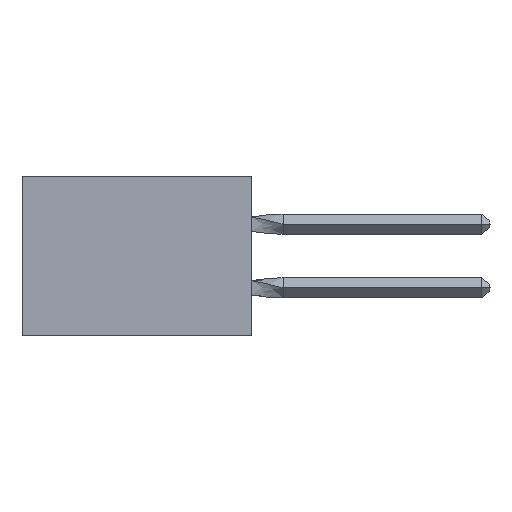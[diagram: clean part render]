
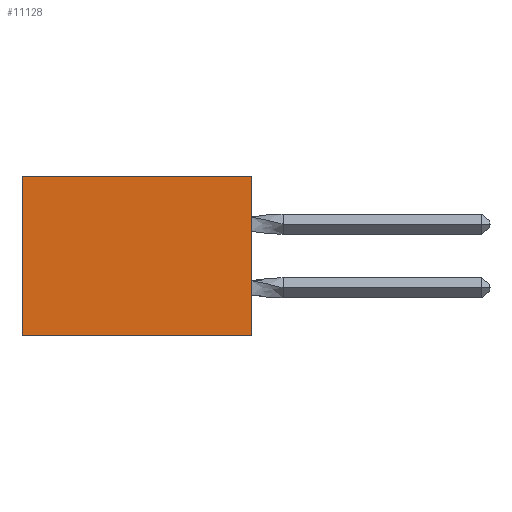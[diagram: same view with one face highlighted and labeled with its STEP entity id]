
A CAD part, left-side view. The second image highlights one B-rep face of the part: STEP entity #11128.
In plain terms, the highlighted planar face has unit normal (-1, 0, 0).
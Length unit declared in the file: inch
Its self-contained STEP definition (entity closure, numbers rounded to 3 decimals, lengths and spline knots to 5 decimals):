
#787 = CARTESIAN_POINT ( 'NONE',  ( 0.305, 0.72, -0.5 ) ) ;
#1518 = CARTESIAN_POINT ( 'NONE',  ( 0.305, 0.72, 0. ) ) ;
#1751 = EDGE_CURVE ( 'NONE', #24773, #32293, #24246, .T. ) ;
#1872 = CARTESIAN_POINT ( 'NONE',  ( 0.305, 0., -0.5 ) ) ;
#1964 = CARTESIAN_POINT ( 'NONE',  ( 0.305, 0., -0.5 ) ) ;
#2946 = CARTESIAN_POINT ( 'NONE',  ( 0.305, 0., 0. ) ) ;
#3001 = EDGE_CURVE ( 'NONE', #18460, #26884, #5622, .T. ) ;
#5005 = CARTESIAN_POINT ( 'NONE',  ( 0.305, 0., 0. ) ) ;
#5140 = FACE_OUTER_BOUND ( 'NONE', #13276, .T. ) ;
#5622 = LINE ( 'NONE', #2946, #24596 ) ;
#5819 = EDGE_CURVE ( 'NONE', #26884, #32293, #26510, .T. ) ;
#8631 = ORIENTED_EDGE ( 'NONE', *, *, #1751, .F. ) ;
#11128 = ADVANCED_FACE ( 'NONE', ( #5140 ), #12002, .F. ) ;
#12002 = PLANE ( 'NONE',  #22472 ) ;
#12854 = DIRECTION ( 'NONE',  ( 0., 1., 0. ) ) ;
#13276 = EDGE_LOOP ( 'NONE', ( #14038, #8631, #29816, #23119 ) ) ;
#14038 = ORIENTED_EDGE ( 'NONE', *, *, #5819, .T. ) ;
#14387 = VECTOR ( 'NONE', #27925, 39.37008 ) ;
#14745 = VECTOR ( 'NONE', #18538, 39.37008 ) ;
#17180 = DIRECTION ( 'NONE',  ( 0., 0., -1. ) ) ;
#18460 = VERTEX_POINT ( 'NONE', #5005 ) ;
#18538 = DIRECTION ( 'NONE',  ( 0., 0., -1. ) ) ;
#19913 = CARTESIAN_POINT ( 'NONE',  ( 0.305, 0., -0.5 ) ) ;
#20126 = CARTESIAN_POINT ( 'NONE',  ( 0.305, 0.72, -0.5 ) ) ;
#22472 = AXIS2_PLACEMENT_3D ( 'NONE', #1872, #29611, #17180 ) ;
#22620 = CARTESIAN_POINT ( 'NONE',  ( 0.305, 0., -0.5 ) ) ;
#23119 = ORIENTED_EDGE ( 'NONE', *, *, #3001, .T. ) ;
#24208 = LINE ( 'NONE', #19913, #14387 ) ;
#24246 = LINE ( 'NONE', #22620, #26993 ) ;
#24596 = VECTOR ( 'NONE', #25786, 39.37008 ) ;
#24773 = VERTEX_POINT ( 'NONE', #1964 ) ;
#25786 = DIRECTION ( 'NONE',  ( 0., 1., 0. ) ) ;
#25923 = EDGE_CURVE ( 'NONE', #18460, #24773, #24208, .T. ) ;
#26510 = LINE ( 'NONE', #787, #14745 ) ;
#26884 = VERTEX_POINT ( 'NONE', #1518 ) ;
#26993 = VECTOR ( 'NONE', #12854, 39.37008 ) ;
#27925 = DIRECTION ( 'NONE',  ( 0., 0., -1. ) ) ;
#29611 = DIRECTION ( 'NONE',  ( 1., 0., 0. ) ) ;
#29816 = ORIENTED_EDGE ( 'NONE', *, *, #25923, .F. ) ;
#32293 = VERTEX_POINT ( 'NONE', #20126 ) ;
